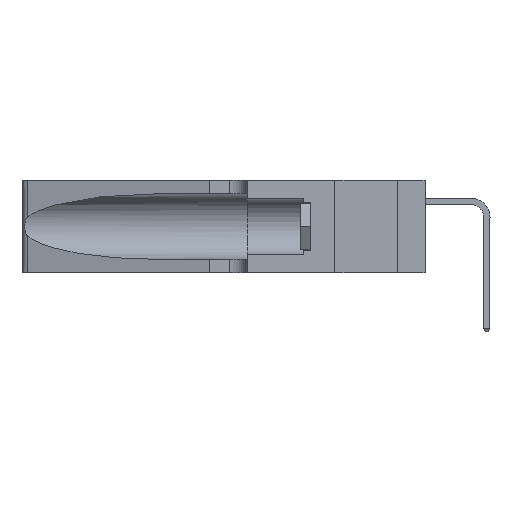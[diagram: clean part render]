
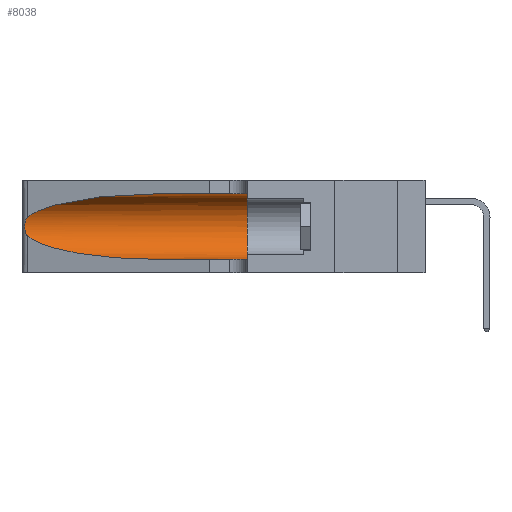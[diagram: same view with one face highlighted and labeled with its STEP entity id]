
A CAD part, left-side view. The second image highlights one B-rep face of the part: STEP entity #8038.
In plain terms, the highlighted cylindrical face has radius 3.308 mm (diameter 6.617 mm), a partial arc.
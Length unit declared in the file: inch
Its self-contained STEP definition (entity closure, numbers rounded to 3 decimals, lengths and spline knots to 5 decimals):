
#588 = CARTESIAN_POINT ( 'NONE',  ( 0.26075, 1.23896, 0.19203 ) ) ;
#616 = VERTEX_POINT ( 'NONE', #10422 ) ;
#1273 = VERTEX_POINT ( 'NONE', #7672 ) ;
#1445 = CARTESIAN_POINT ( 'NONE',  ( 0.25487, 1.22718, 0.14631 ) ) ;
#1470 = CARTESIAN_POINT ( 'NONE',  ( 0.2373, 1.15595, 0.28018 ) ) ;
#2297 = CARTESIAN_POINT ( 'NONE',  ( 0.1305, 0.35, 0.05475 ) ) ;
#2430 = CARTESIAN_POINT ( 'NONE',  ( 0.25555, 1.22994, 0.2215 ) ) ;
#2513 = CARTESIAN_POINT ( 'NONE',  ( 0.26017, 1.23833, 0.17102 ) ) ;
#2676 = EDGE_CURVE ( 'NONE', #616, #23779, #14399, .T. ) ;
#2904 = ORIENTED_EDGE ( 'NONE', *, *, #17123, .T. ) ;
#3128 = CYLINDRICAL_SURFACE ( 'NONE', #5027, 0.13025 ) ;
#4191 = VECTOR ( 'NONE', #14789, 39.37008 ) ;
#4292 = EDGE_CURVE ( 'NONE', #19721, #13782, #10571, .T. ) ;
#4502 = CARTESIAN_POINT ( 'NONE',  ( 0.25789, 1.23486, 0.15765 ) ) ;
#5027 = AXIS2_PLACEMENT_3D ( 'NONE', #20863, #17055, #9471 ) ;
#5247 = CARTESIAN_POINT ( 'NONE',  ( 0.1305, 1.61858, 0.05475 ) ) ;
#5932 = LINE ( 'NONE', #12703, #15526 ) ;
#5938 = EDGE_CURVE ( 'NONE', #7765, #23779, #10969, .T. ) ;
#6154 = ORIENTED_EDGE ( 'NONE', *, *, #17110, .T. ) ;
#6405 = CARTESIAN_POINT ( 'NONE',  ( 0.25555, 1.22993, 0.14849 ) ) ;
#7138 = ORIENTED_EDGE ( 'NONE', *, *, #2676, .T. ) ;
#7148 = CARTESIAN_POINT ( 'NONE',  ( 0.2373, 1.15595, 0.08982 ) ) ;
#7672 = CARTESIAN_POINT ( 'NONE',  ( 0.1305, 0.72297, 0.31525 ) ) ;
#7765 = VERTEX_POINT ( 'NONE', #21528 ) ;
#8038 = ADVANCED_FACE ( 'NONE', ( #13339 ), #3128, .F. ) ;
#8264 = CARTESIAN_POINT ( 'NONE',  ( 0.25487, 1.22718, 0.22369 ) ) ;
#8936 =( BOUNDED_CURVE ( )  B_SPLINE_CURVE ( 3, ( #16662, #7148, #22360, #11002 ),
 .UNSPECIFIED., .F., .F. ) 
 B_SPLINE_CURVE_WITH_KNOTS ( ( 4, 4 ),
 ( 3.44316, 4.71239 ),
 .UNSPECIFIED. ) 
 CURVE ( )  GEOMETRIC_REPRESENTATION_ITEM ( )  RATIONAL_B_SPLINE_CURVE ( ( 1., 0.87, 0.87, 1. ) ) 
 REPRESENTATION_ITEM ( '' )  );
#9046 = ORIENTED_EDGE ( 'NONE', *, *, #5938, .F. ) ;
#9471 = DIRECTION ( 'NONE',  ( 0., 0., -1. ) ) ;
#9483 = ORIENTED_EDGE ( 'NONE', *, *, #14463, .F. ) ;
#10203 = CARTESIAN_POINT ( 'NONE',  ( 0.25787, 1.23484, 0.2124 ) ) ;
#10422 = CARTESIAN_POINT ( 'NONE',  ( 0.1305, 0.72297, 0.05475 ) ) ;
#10571 = B_SPLINE_CURVE_WITH_KNOTS ( 'NONE', 3,
 ( #8264, #2430, #17753, #10203, #23443, #12104, #588, #14036, #2513, #15952, #4502, #17841, #6405, #19754 ),
 .UNSPECIFIED., .F., .F.,
 ( 4, 2, 2, 2, 2, 2, 4 ),
 ( 0., 0.00027, 0.00053, 0.00107, 0.0016, 0.00187, 0.00214 ),
 .UNSPECIFIED. ) ;
#10665 = DIRECTION ( 'NONE',  ( 0., 1., 0. ) ) ;
#10969 = CIRCLE ( 'NONE', #11849, 0.13025 ) ;
#11002 = CARTESIAN_POINT ( 'NONE',  ( 0.1305, 0.72297, 0.05475 ) ) ;
#11086 = CARTESIAN_POINT ( 'NONE',  ( 0.18966, 0.96281, 0.31525 ) ) ;
#11849 = AXIS2_PLACEMENT_3D ( 'NONE', #22029, #10665, #23904 ) ;
#12104 = CARTESIAN_POINT ( 'NONE',  ( 0.26018, 1.23835, 0.19895 ) ) ;
#12703 = CARTESIAN_POINT ( 'NONE',  ( 0.1305, 1.61858, 0.31525 ) ) ;
#13339 = FACE_OUTER_BOUND ( 'NONE', #18571, .T. ) ;
#13729 = ORIENTED_EDGE ( 'NONE', *, *, #4292, .T. ) ;
#13782 = VERTEX_POINT ( 'NONE', #1445 ) ;
#14036 = CARTESIAN_POINT ( 'NONE',  ( 0.26075, 1.23896, 0.178 ) ) ;
#14399 = LINE ( 'NONE', #5247, #4191 ) ;
#14463 = EDGE_CURVE ( 'NONE', #1273, #7765, #5932, .T. ) ;
#14633 = DIRECTION ( 'NONE',  ( 0., -1., 0. ) ) ;
#14789 = DIRECTION ( 'NONE',  ( 0., -1., 0. ) ) ;
#14924 = CARTESIAN_POINT ( 'NONE',  ( 0.25487, 1.22718, 0.22369 ) ) ;
#15526 = VECTOR ( 'NONE', #14633, 39.37008 ) ;
#15952 = CARTESIAN_POINT ( 'NONE',  ( 0.25856, 1.23593, 0.16098 ) ) ;
#16662 = CARTESIAN_POINT ( 'NONE',  ( 0.25487, 1.22718, 0.14631 ) ) ;
#17055 = DIRECTION ( 'NONE',  ( 0., -1., 0. ) ) ;
#17110 = EDGE_CURVE ( 'NONE', #13782, #616, #8936, .T. ) ;
#17123 = EDGE_CURVE ( 'NONE', #1273, #19721, #17785, .T. ) ;
#17753 = CARTESIAN_POINT ( 'NONE',  ( 0.25639, 1.23184, 0.21858 ) ) ;
#17785 =( BOUNDED_CURVE ( )  B_SPLINE_CURVE ( 3, ( #24317, #11086, #1470, #14924 ),
 .UNSPECIFIED., .F., .F. ) 
 B_SPLINE_CURVE_WITH_KNOTS ( ( 4, 4 ),
 ( 1.5708, 2.84003 ),
 .UNSPECIFIED. ) 
 CURVE ( )  GEOMETRIC_REPRESENTATION_ITEM ( )  RATIONAL_B_SPLINE_CURVE ( ( 1., 0.87, 0.87, 1. ) ) 
 REPRESENTATION_ITEM ( '' )  );
#17841 = CARTESIAN_POINT ( 'NONE',  ( 0.25639, 1.23186, 0.15144 ) ) ;
#18571 = EDGE_LOOP ( 'NONE', ( #2904, #13729, #6154, #7138, #9046, #9483 ) ) ;
#19721 = VERTEX_POINT ( 'NONE', #21684 ) ;
#19754 = CARTESIAN_POINT ( 'NONE',  ( 0.25487, 1.22718, 0.14631 ) ) ;
#20863 = CARTESIAN_POINT ( 'NONE',  ( 0.1305, 1.61858, 0.185 ) ) ;
#21528 = CARTESIAN_POINT ( 'NONE',  ( 0.1305, 0.35, 0.31525 ) ) ;
#21684 = CARTESIAN_POINT ( 'NONE',  ( 0.25487, 1.22718, 0.22369 ) ) ;
#22029 = CARTESIAN_POINT ( 'NONE',  ( 0.1305, 0.35, 0.185 ) ) ;
#22360 = CARTESIAN_POINT ( 'NONE',  ( 0.18966, 0.96281, 0.05475 ) ) ;
#23443 = CARTESIAN_POINT ( 'NONE',  ( 0.25854, 1.2359, 0.20912 ) ) ;
#23779 = VERTEX_POINT ( 'NONE', #2297 ) ;
#23904 = DIRECTION ( 'NONE',  ( 0., 0., 1. ) ) ;
#24317 = CARTESIAN_POINT ( 'NONE',  ( 0.1305, 0.72297, 0.31525 ) ) ;
